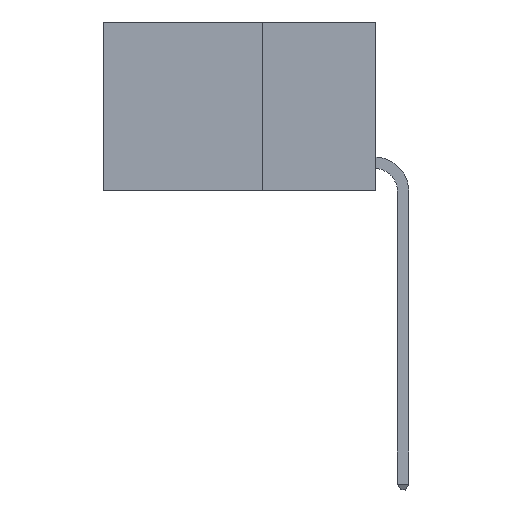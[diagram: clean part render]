
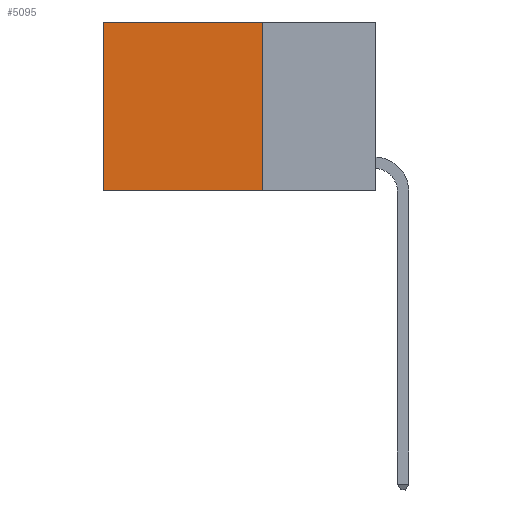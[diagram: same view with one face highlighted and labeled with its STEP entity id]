
A CAD part, left-side view. The second image highlights one B-rep face of the part: STEP entity #5095.
In plain terms, the highlighted planar face has unit normal (-1, 0, 0).
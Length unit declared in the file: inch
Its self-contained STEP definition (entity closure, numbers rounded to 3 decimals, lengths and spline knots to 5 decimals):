
#1084 = ORIENTED_EDGE ( 'NONE', *, *, #2370, .F. ) ;
#1157 = PLANE ( 'NONE',  #3338 ) ;
#1467 = LINE ( 'NONE', #2843, #12092 ) ;
#1938 = EDGE_LOOP ( 'NONE', ( #5665, #4600, #1084, #15636 ) ) ;
#2370 = EDGE_CURVE ( 'NONE', #5188, #3245, #18641, .T. ) ;
#2441 = FACE_OUTER_BOUND ( 'NONE', #1938, .T. ) ;
#2694 = DIRECTION ( 'NONE',  ( 1., 0., 0. ) ) ;
#2821 = CARTESIAN_POINT ( 'NONE',  ( 0.2625, 0.25, -0.37 ) ) ;
#2843 = CARTESIAN_POINT ( 'NONE',  ( 0.2625, 0.25, -0.37 ) ) ;
#3245 = VERTEX_POINT ( 'NONE', #2821 ) ;
#3338 = AXIS2_PLACEMENT_3D ( 'NONE', #11715, #2694, #13183 ) ;
#4600 = ORIENTED_EDGE ( 'NONE', *, *, #9590, .F. ) ;
#5095 = ADVANCED_FACE ( 'NONE', ( #2441 ), #1157, .F. ) ;
#5188 = VERTEX_POINT ( 'NONE', #8930 ) ;
#5665 = ORIENTED_EDGE ( 'NONE', *, *, #11227, .T. ) ;
#7113 = VECTOR ( 'NONE', #12777, 39.37008 ) ;
#8930 = CARTESIAN_POINT ( 'NONE',  ( 0.2625, 0.25, 0. ) ) ;
#8975 = CARTESIAN_POINT ( 'NONE',  ( 0.2625, 0.6, 0. ) ) ;
#9590 = EDGE_CURVE ( 'NONE', #3245, #17595, #1467, .T. ) ;
#10740 = EDGE_CURVE ( 'NONE', #5188, #11996, #15410, .T. ) ;
#11227 = EDGE_CURVE ( 'NONE', #11996, #17595, #15394, .T. ) ;
#11715 = CARTESIAN_POINT ( 'NONE',  ( 0.2625, 0.25, 0. ) ) ;
#11996 = VERTEX_POINT ( 'NONE', #8975 ) ;
#12092 = VECTOR ( 'NONE', #14749, 39.37008 ) ;
#12517 = DIRECTION ( 'NONE',  ( 0., 0., -1. ) ) ;
#12777 = DIRECTION ( 'NONE',  ( 0., 0., -1. ) ) ;
#13183 = DIRECTION ( 'NONE',  ( 0., 0., -1. ) ) ;
#13340 = CARTESIAN_POINT ( 'NONE',  ( 0.2625, 0.25, 0. ) ) ;
#14410 = CARTESIAN_POINT ( 'NONE',  ( 0.2625, 0.25, 0. ) ) ;
#14749 = DIRECTION ( 'NONE',  ( 0., 1., 0. ) ) ;
#14975 = VECTOR ( 'NONE', #15816, 39.37008 ) ;
#15394 = LINE ( 'NONE', #16733, #18272 ) ;
#15410 = LINE ( 'NONE', #14410, #14975 ) ;
#15636 = ORIENTED_EDGE ( 'NONE', *, *, #10740, .T. ) ;
#15816 = DIRECTION ( 'NONE',  ( 0., 1., 0. ) ) ;
#16733 = CARTESIAN_POINT ( 'NONE',  ( 0.2625, 0.6, 0. ) ) ;
#17595 = VERTEX_POINT ( 'NONE', #18448 ) ;
#18272 = VECTOR ( 'NONE', #12517, 39.37008 ) ;
#18448 = CARTESIAN_POINT ( 'NONE',  ( 0.2625, 0.6, -0.37 ) ) ;
#18641 = LINE ( 'NONE', #13340, #7113 ) ;
